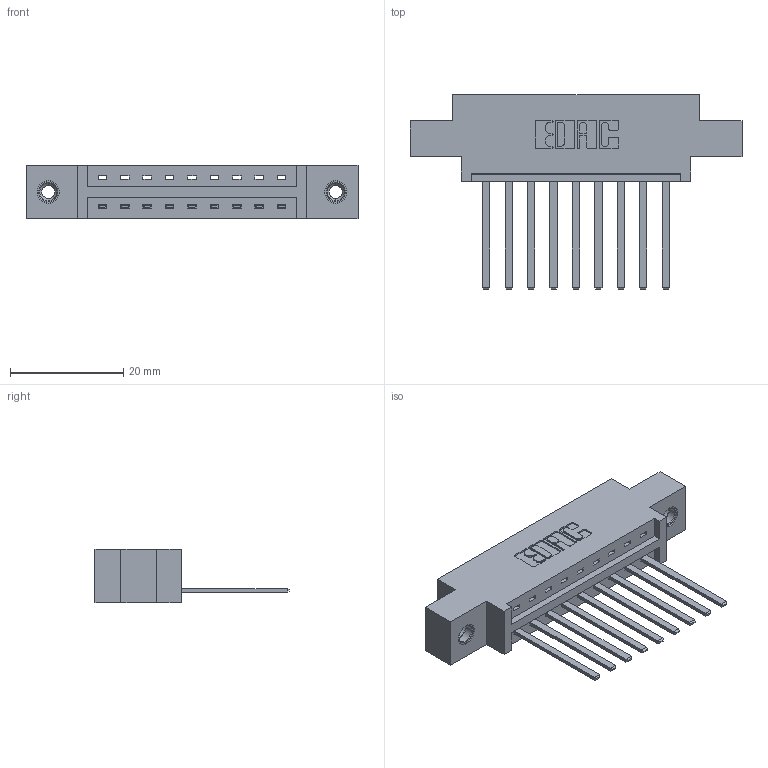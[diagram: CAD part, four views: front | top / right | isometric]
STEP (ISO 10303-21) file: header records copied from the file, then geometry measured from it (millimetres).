
FILE_DESCRIPTION (( 'STEP AP203' ), '1' );
FILE_NAME ('337-009-544-608.STEP', '2018-08-03T23:03:40', ( '' ), ( '' ), 'SwSTEP 2.0', 'SolidWorks 2016', '' );
FILE_SCHEMA (( 'CONFIG_CONTROL_DESIGN' ));
Length unit declared in the file: inch
Products named in the file (4): 337-009-544-608; 337 Part_0.170 Offset - 0.156 Dia-TI; 345-292-001_345-293-144; 345-250-001_345-250-003-102
Assembly tree (12 placements, depth 2):
  337-009-544-608
    337 Part_0.170 Offset - 0.156 Dia-TI
    345-292-001_345-293-144  x9
    345-250-001_345-250-003-102  x2
Bounding box: 58.67 x 34.3 x 9.4 mm (x, y, z)
Volume: 5665.4 mm3; surface area: 6140.2 mm2
Topology: 12 solids, 12 shells, 682 faces, 1989 edges, 1306 vertices
Faces by surface type: plane 484, cylinder 182, cone 12, torus 4
Entity records: 12092 total; most frequent: CARTESIAN_POINT 2084, ORIENTED_EDGE 2022, DIRECTION 1851, EDGE_CURVE 1011, LINE 867, VECTOR 867, VERTEX_POINT 668, AXIS2_PLACEMENT_3D 492
